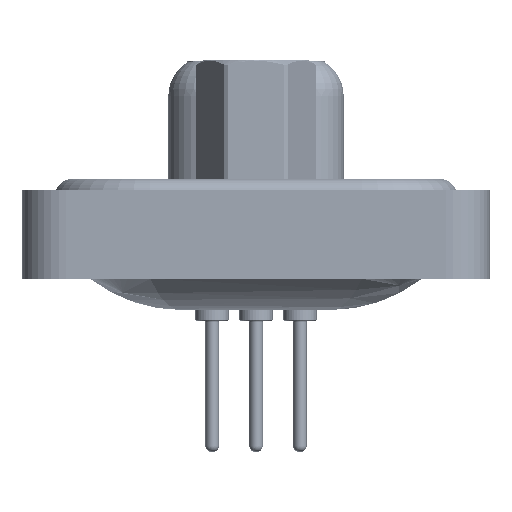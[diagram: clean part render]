
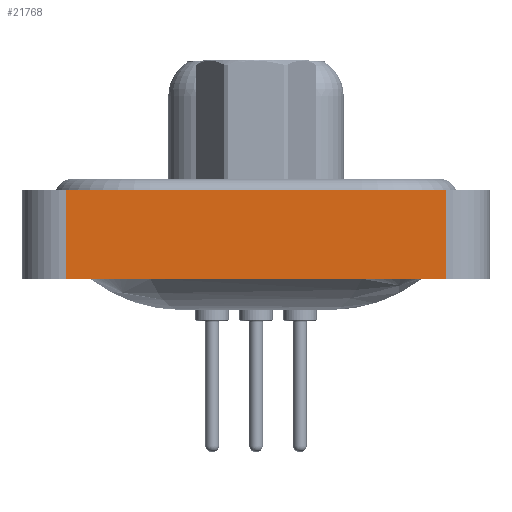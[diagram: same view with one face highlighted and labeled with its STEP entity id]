
A CAD part, left-side view. The second image highlights one B-rep face of the part: STEP entity #21768.
In plain terms, the highlighted planar face has unit normal (-1, 0, 0).
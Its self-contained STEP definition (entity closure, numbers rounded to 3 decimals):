
#2728 = VECTOR ( 'NONE', #27248, 1000. ) ;
#4097 = CARTESIAN_POINT ( 'NONE',  ( -7.35, 8.55, -3.6 ) ) ;
#4551 = EDGE_CURVE ( 'NONE', #13376, #21661, #10809, .T. ) ;
#4874 = VERTEX_POINT ( 'NONE', #10581 ) ;
#5186 = ORIENTED_EDGE ( 'NONE', *, *, #4551, .F. ) ;
#5191 = LINE ( 'NONE', #27564, #37496 ) ;
#6372 = DIRECTION ( 'NONE',  ( 0., -1., 0. ) ) ;
#7371 = CARTESIAN_POINT ( 'NONE',  ( -7.35, -8.55, 0.4 ) ) ;
#10034 = DIRECTION ( 'NONE',  ( 0., 0., 1. ) ) ;
#10271 = AXIS2_PLACEMENT_3D ( 'NONE', #32019, #38037, #19962 ) ;
#10581 = CARTESIAN_POINT ( 'NONE',  ( -7.35, -8.55, 0.4 ) ) ;
#10809 = LINE ( 'NONE', #24053, #2728 ) ;
#12786 = ORIENTED_EDGE ( 'NONE', *, *, #21575, .T. ) ;
#13376 = VERTEX_POINT ( 'NONE', #4097 ) ;
#15863 = VECTOR ( 'NONE', #28536, 1000. ) ;
#16905 = PLANE ( 'NONE',  #10271 ) ;
#19962 = DIRECTION ( 'NONE',  ( 0., 0., 1. ) ) ;
#21428 = VECTOR ( 'NONE', #10034, 1000. ) ;
#21575 = EDGE_CURVE ( 'NONE', #24941, #4874, #22359, .T. ) ;
#21661 = VERTEX_POINT ( 'NONE', #28537 ) ;
#21768 = ADVANCED_FACE ( 'NONE', ( #31873 ), #16905, .T. ) ;
#22063 = CARTESIAN_POINT ( 'NONE',  ( -7.35, -8.55, -3.6 ) ) ;
#22309 = ORIENTED_EDGE ( 'NONE', *, *, #28010, .F. ) ;
#22359 = LINE ( 'NONE', #22063, #21428 ) ;
#24053 = CARTESIAN_POINT ( 'NONE',  ( -7.35, 8.55, -3.6 ) ) ;
#24591 = ORIENTED_EDGE ( 'NONE', *, *, #32560, .T. ) ;
#24941 = VERTEX_POINT ( 'NONE', #28746 ) ;
#25771 = LINE ( 'NONE', #7371, #15863 ) ;
#26816 = EDGE_LOOP ( 'NONE', ( #12786, #22309, #5186, #24591 ) ) ;
#27248 = DIRECTION ( 'NONE',  ( 0., 0., 1. ) ) ;
#27564 = CARTESIAN_POINT ( 'NONE',  ( -7.35, -8.55, -3.6 ) ) ;
#28010 = EDGE_CURVE ( 'NONE', #21661, #4874, #25771, .T. ) ;
#28536 = DIRECTION ( 'NONE',  ( 0., -1., 0. ) ) ;
#28537 = CARTESIAN_POINT ( 'NONE',  ( -7.35, 8.55, 0.4 ) ) ;
#28746 = CARTESIAN_POINT ( 'NONE',  ( -7.35, -8.55, -3.6 ) ) ;
#31873 = FACE_OUTER_BOUND ( 'NONE', #26816, .T. ) ;
#32019 = CARTESIAN_POINT ( 'NONE',  ( -7.35, -8.55, -3.6 ) ) ;
#32560 = EDGE_CURVE ( 'NONE', #13376, #24941, #5191, .T. ) ;
#37496 = VECTOR ( 'NONE', #6372, 1000. ) ;
#38037 = DIRECTION ( 'NONE',  ( -1., 0., 0. ) ) ;
